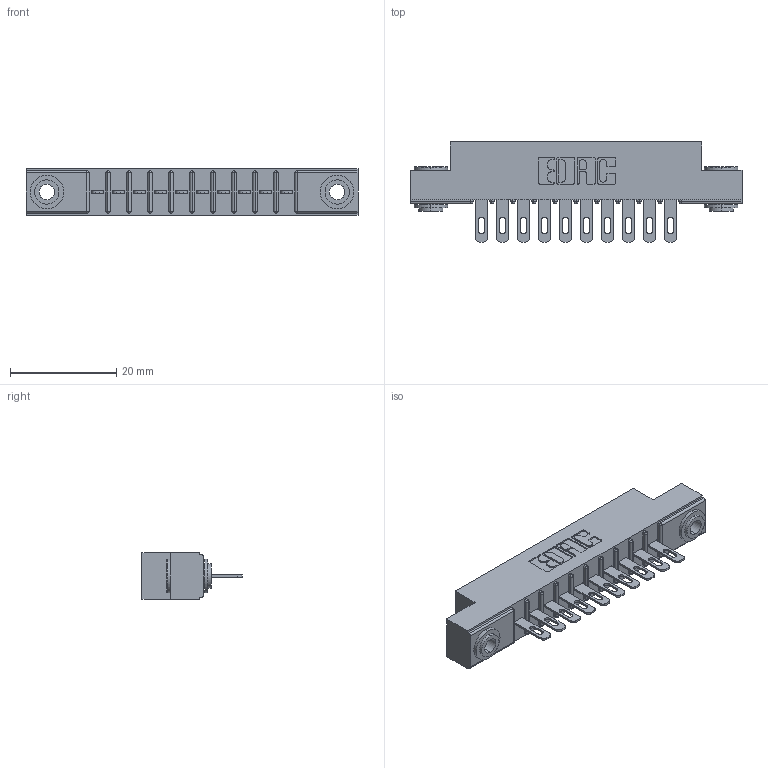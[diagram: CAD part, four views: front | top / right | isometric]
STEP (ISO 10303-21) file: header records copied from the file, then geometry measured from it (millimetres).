
FILE_DESCRIPTION (( 'STEP AP203' ), '1' );
FILE_NAME ('356-010-500-103.STEP', '2018-07-31T06:56:01', ( '' ), ( '' ), 'SwSTEP 2.0', 'SolidWorks 2016', '' );
FILE_SCHEMA (( 'CONFIG_CONTROL_DESIGN' ));
Length unit declared in the file: inch
Products named in the file (4): 356-010-500-103; 306 Part_.156 Dia; 306-290-001_100; 345-250-002_345-250-002-102
Assembly tree (13 placements, depth 2):
  356-010-500-103
    306 Part_.156 Dia
    306-290-001_100  x10
    345-250-002_345-250-002-102  x2
Bounding box: 62.64 x 18.87 x 8.71 mm (x, y, z)
Volume: 4260.4 mm3; surface area: 6342 mm2
Topology: 13 solids, 13 shells, 928 faces, 2578 edges, 1660 vertices
Faces by surface type: plane 592, cylinder 288, sphere 40, cone 8
Entity records: 14700 total; most frequent: CARTESIAN_POINT 2442, DIRECTION 2426, ORIENTED_EDGE 2408, EDGE_CURVE 1204, VECTOR 914, LINE 914, VERTEX_POINT 772, AXIS2_PLACEMENT_3D 756
